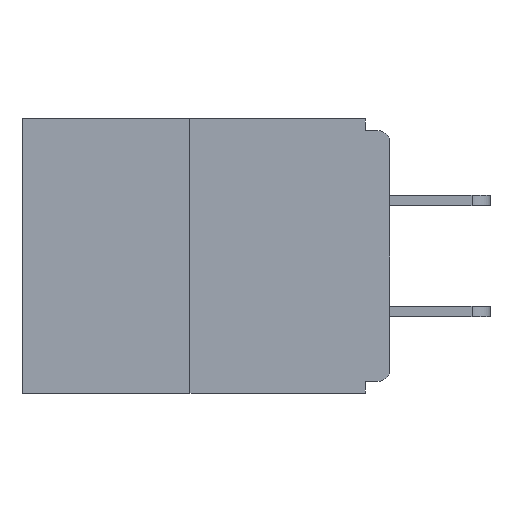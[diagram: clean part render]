
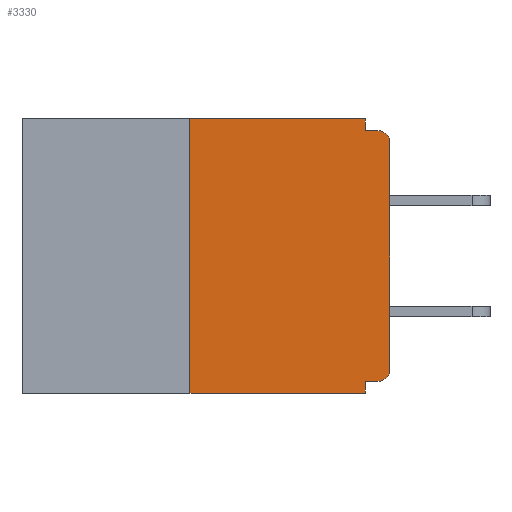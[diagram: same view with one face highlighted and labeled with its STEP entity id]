
A CAD part, left-side view. The second image highlights one B-rep face of the part: STEP entity #3330.
In plain terms, the highlighted planar face has unit normal (-1, 0, 0).
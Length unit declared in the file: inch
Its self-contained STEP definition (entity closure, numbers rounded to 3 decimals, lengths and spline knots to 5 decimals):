
#215 = ORIENTED_EDGE ( 'NONE', *, *, #9783, .F. ) ;
#364 = VERTEX_POINT ( 'NONE', #5657 ) ;
#505 = ORIENTED_EDGE ( 'NONE', *, *, #19535, .F. ) ;
#952 = CARTESIAN_POINT ( 'NONE',  ( 0., 0.015, -0.313 ) ) ;
#1041 = DIRECTION ( 'NONE',  ( 0., -1., 0. ) ) ;
#1500 = FACE_OUTER_BOUND ( 'NONE', #17245, .T. ) ;
#1715 = VERTEX_POINT ( 'NONE', #2862 ) ;
#1742 = VECTOR ( 'NONE', #10300, 39.37008 ) ;
#1801 = VECTOR ( 'NONE', #1041, 39.37008 ) ;
#2408 = VECTOR ( 'NONE', #7430, 39.37008 ) ;
#2430 = ORIENTED_EDGE ( 'NONE', *, *, #15130, .T. ) ;
#2546 = EDGE_CURVE ( 'NONE', #5079, #19411, #3038, .T. ) ;
#2862 = CARTESIAN_POINT ( 'NONE',  ( 0., 0.25, -0.343 ) ) ;
#2918 = AXIS2_PLACEMENT_3D ( 'NONE', #14141, #8058, #9598 ) ;
#2999 = LINE ( 'NONE', #6008, #3491 ) ;
#3038 = LINE ( 'NONE', #13792, #19569 ) ;
#3139 = CARTESIAN_POINT ( 'NONE',  ( 0., 0.015, -0.03 ) ) ;
#3330 = ADVANCED_FACE ( 'NONE', ( #1500 ), #6406, .F. ) ;
#3491 = VECTOR ( 'NONE', #16728, 39.37008 ) ;
#3884 = ORIENTED_EDGE ( 'NONE', *, *, #9014, .F. ) ;
#3942 = CARTESIAN_POINT ( 'NONE',  ( 0., 0.031, 0. ) ) ;
#4258 = CIRCLE ( 'NONE', #12944, 0.015 ) ;
#4559 = DIRECTION ( 'NONE',  ( 0., -1., 0. ) ) ;
#4576 = CARTESIAN_POINT ( 'NONE',  ( 0., 0.031, -0.328 ) ) ;
#5079 = VERTEX_POINT ( 'NONE', #8290 ) ;
#5288 = DIRECTION ( 'NONE',  ( -1., 0., 0. ) ) ;
#5411 = EDGE_CURVE ( 'NONE', #17236, #15691, #14656, .T. ) ;
#5657 = CARTESIAN_POINT ( 'NONE',  ( 0., 0.015, -0.015 ) ) ;
#6008 = CARTESIAN_POINT ( 'NONE',  ( 0., 0., -0.328 ) ) ;
#6116 = CIRCLE ( 'NONE', #18609, 0.015 ) ;
#6281 = LINE ( 'NONE', #8780, #1742 ) ;
#6406 = PLANE ( 'NONE',  #2918 ) ;
#6732 = DIRECTION ( 'NONE',  ( 0., 0., -1. ) ) ;
#7368 = CARTESIAN_POINT ( 'NONE',  ( 0., 0., 0. ) ) ;
#7430 = DIRECTION ( 'NONE',  ( 0., 0., 1. ) ) ;
#7637 = DIRECTION ( 'NONE',  ( 0., -1., 0. ) ) ;
#8058 = DIRECTION ( 'NONE',  ( 1., 0., 0. ) ) ;
#8286 = EDGE_CURVE ( 'NONE', #18925, #364, #18330, .T. ) ;
#8290 = CARTESIAN_POINT ( 'NONE',  ( 0., 0.25, 0. ) ) ;
#8376 = EDGE_CURVE ( 'NONE', #15691, #364, #6116, .T. ) ;
#8454 = CARTESIAN_POINT ( 'NONE',  ( 0., 0., -0.313 ) ) ;
#8760 = CARTESIAN_POINT ( 'NONE',  ( 0., 0., -0.015 ) ) ;
#8780 = CARTESIAN_POINT ( 'NONE',  ( 0., 0.25, 0. ) ) ;
#9014 = EDGE_CURVE ( 'NONE', #16864, #14584, #2999, .T. ) ;
#9598 = DIRECTION ( 'NONE',  ( 0., 0., -1. ) ) ;
#9665 = ORIENTED_EDGE ( 'NONE', *, *, #11765, .F. ) ;
#9783 = EDGE_CURVE ( 'NONE', #19411, #18925, #10690, .T. ) ;
#9946 = DIRECTION ( 'NONE',  ( 0., 0., -1. ) ) ;
#10300 = DIRECTION ( 'NONE',  ( 0., 0., 1. ) ) ;
#10588 = LINE ( 'NONE', #14517, #18206 ) ;
#10663 = CARTESIAN_POINT ( 'NONE',  ( 0., 0.46, -0.343 ) ) ;
#10690 = LINE ( 'NONE', #3942, #14979 ) ;
#10752 = VERTEX_POINT ( 'NONE', #11321 ) ;
#11321 = CARTESIAN_POINT ( 'NONE',  ( 0., 0.031, -0.343 ) ) ;
#11377 = ORIENTED_EDGE ( 'NONE', *, *, #8376, .T. ) ;
#11591 = CARTESIAN_POINT ( 'NONE',  ( 0., 0.031, 0. ) ) ;
#11765 = EDGE_CURVE ( 'NONE', #14584, #10752, #10588, .T. ) ;
#12944 = AXIS2_PLACEMENT_3D ( 'NONE', #952, #5288, #9946 ) ;
#13144 = CARTESIAN_POINT ( 'NONE',  ( 0., 0.015, -0.328 ) ) ;
#13522 = ORIENTED_EDGE ( 'NONE', *, *, #8286, .F. ) ;
#13792 = CARTESIAN_POINT ( 'NONE',  ( 0., 0.46, 0. ) ) ;
#13825 = ORIENTED_EDGE ( 'NONE', *, *, #16764, .T. ) ;
#13885 = DIRECTION ( 'NONE',  ( -1., 0., 0. ) ) ;
#14141 = CARTESIAN_POINT ( 'NONE',  ( 0., 0.46, 0. ) ) ;
#14457 = ORIENTED_EDGE ( 'NONE', *, *, #5411, .T. ) ;
#14517 = CARTESIAN_POINT ( 'NONE',  ( 0., 0.031, -0.343 ) ) ;
#14584 = VERTEX_POINT ( 'NONE', #4576 ) ;
#14656 = LINE ( 'NONE', #7368, #2408 ) ;
#14699 = DIRECTION ( 'NONE',  ( 0., 0., -1. ) ) ;
#14979 = VECTOR ( 'NONE', #14699, 39.37008 ) ;
#15037 = CARTESIAN_POINT ( 'NONE',  ( 0., 0.031, -0.015 ) ) ;
#15130 = EDGE_CURVE ( 'NONE', #16864, #17236, #4258, .T. ) ;
#15386 = ORIENTED_EDGE ( 'NONE', *, *, #2546, .F. ) ;
#15691 = VERTEX_POINT ( 'NONE', #19186 ) ;
#16439 = LINE ( 'NONE', #10663, #19518 ) ;
#16728 = DIRECTION ( 'NONE',  ( 0., 1., 0. ) ) ;
#16764 = EDGE_CURVE ( 'NONE', #1715, #10752, #16439, .T. ) ;
#16864 = VERTEX_POINT ( 'NONE', #13144 ) ;
#17236 = VERTEX_POINT ( 'NONE', #8454 ) ;
#17245 = EDGE_LOOP ( 'NONE', ( #15386, #505, #13825, #9665, #3884, #2430, #14457, #11377, #13522, #215 ) ) ;
#18206 = VECTOR ( 'NONE', #6732, 39.37008 ) ;
#18330 = LINE ( 'NONE', #8760, #1801 ) ;
#18556 = DIRECTION ( 'NONE',  ( 0., 0., -1. ) ) ;
#18609 = AXIS2_PLACEMENT_3D ( 'NONE', #3139, #13885, #18556 ) ;
#18925 = VERTEX_POINT ( 'NONE', #15037 ) ;
#19186 = CARTESIAN_POINT ( 'NONE',  ( 0., 0., -0.03 ) ) ;
#19411 = VERTEX_POINT ( 'NONE', #11591 ) ;
#19518 = VECTOR ( 'NONE', #7637, 39.37008 ) ;
#19535 = EDGE_CURVE ( 'NONE', #1715, #5079, #6281, .T. ) ;
#19569 = VECTOR ( 'NONE', #4559, 39.37008 ) ;
